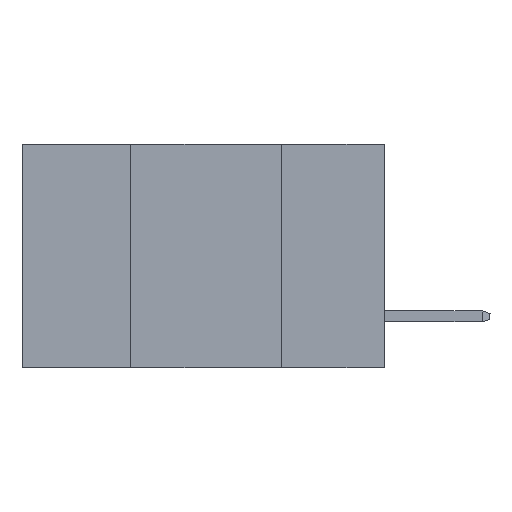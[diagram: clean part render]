
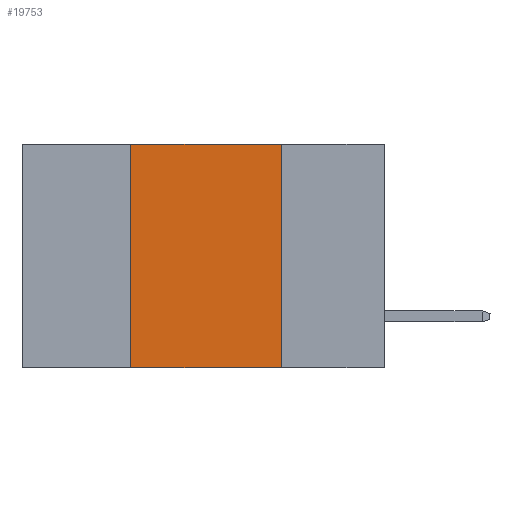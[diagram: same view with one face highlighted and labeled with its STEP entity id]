
A CAD part, left-side view. The second image highlights one B-rep face of the part: STEP entity #19753.
In plain terms, the highlighted planar face has unit normal (-1, 0, 0).
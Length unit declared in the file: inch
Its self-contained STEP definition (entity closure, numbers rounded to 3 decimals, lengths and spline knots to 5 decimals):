
#685 = LINE ( 'NONE', #3577, #20446 ) ;
#706 = CARTESIAN_POINT ( 'NONE',  ( 0., 0.6, 0. ) ) ;
#1123 = CARTESIAN_POINT ( 'NONE',  ( 0., 0.6, 0. ) ) ;
#1249 = VECTOR ( 'NONE', #13911, 39.37008 ) ;
#1708 = DIRECTION ( 'NONE',  ( 0., -1., 0. ) ) ;
#1768 = VECTOR ( 'NONE', #11122, 39.37008 ) ;
#2096 = VERTEX_POINT ( 'NONE', #6848 ) ;
#3577 = CARTESIAN_POINT ( 'NONE',  ( 0., 0.17, -0.37 ) ) ;
#4814 = CARTESIAN_POINT ( 'NONE',  ( 0., 0.17, 0. ) ) ;
#6848 = CARTESIAN_POINT ( 'NONE',  ( 0., 0.42, -0.37 ) ) ;
#6987 = LINE ( 'NONE', #23214, #1249 ) ;
#7388 = ORIENTED_EDGE ( 'NONE', *, *, #24595, .F. ) ;
#7963 = ORIENTED_EDGE ( 'NONE', *, *, #11221, .F. ) ;
#8130 = EDGE_CURVE ( 'NONE', #8196, #23683, #18498, .T. ) ;
#8196 = VERTEX_POINT ( 'NONE', #23898 ) ;
#10422 = DIRECTION ( 'NONE',  ( 0., 0., -1. ) ) ;
#11122 = DIRECTION ( 'NONE',  ( 0., -1., 0. ) ) ;
#11194 = VERTEX_POINT ( 'NONE', #23132 ) ;
#11221 = EDGE_CURVE ( 'NONE', #2096, #8196, #6987, .T. ) ;
#11814 = FACE_OUTER_BOUND ( 'NONE', #15667, .T. ) ;
#13911 = DIRECTION ( 'NONE',  ( 0., 0., 1. ) ) ;
#15667 = EDGE_LOOP ( 'NONE', ( #7388, #17558, #7963, #18138 ) ) ;
#17110 = LINE ( 'NONE', #20550, #1768 ) ;
#17558 = ORIENTED_EDGE ( 'NONE', *, *, #8130, .F. ) ;
#18138 = ORIENTED_EDGE ( 'NONE', *, *, #21801, .T. ) ;
#18498 = LINE ( 'NONE', #1123, #23444 ) ;
#18870 = DIRECTION ( 'NONE',  ( 0., 0., -1. ) ) ;
#19753 = ADVANCED_FACE ( 'NONE', ( #11814 ), #19875, .F. ) ;
#19875 = PLANE ( 'NONE',  #23073 ) ;
#20446 = VECTOR ( 'NONE', #18870, 39.37008 ) ;
#20550 = CARTESIAN_POINT ( 'NONE',  ( 0., 0.6, -0.37 ) ) ;
#21744 = DIRECTION ( 'NONE',  ( 1., 0., 0. ) ) ;
#21801 = EDGE_CURVE ( 'NONE', #2096, #11194, #17110, .T. ) ;
#23073 = AXIS2_PLACEMENT_3D ( 'NONE', #706, #21744, #10422 ) ;
#23132 = CARTESIAN_POINT ( 'NONE',  ( 0., 0.17, -0.37 ) ) ;
#23214 = CARTESIAN_POINT ( 'NONE',  ( 0., 0.42, -0.37 ) ) ;
#23444 = VECTOR ( 'NONE', #1708, 39.37008 ) ;
#23683 = VERTEX_POINT ( 'NONE', #4814 ) ;
#23898 = CARTESIAN_POINT ( 'NONE',  ( 0., 0.42, 0. ) ) ;
#24595 = EDGE_CURVE ( 'NONE', #23683, #11194, #685, .T. ) ;
